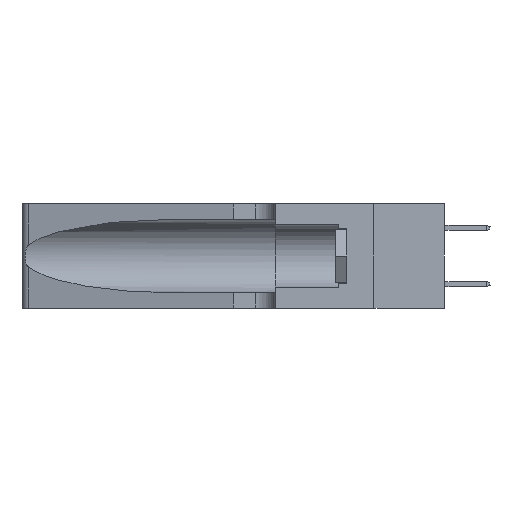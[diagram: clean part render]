
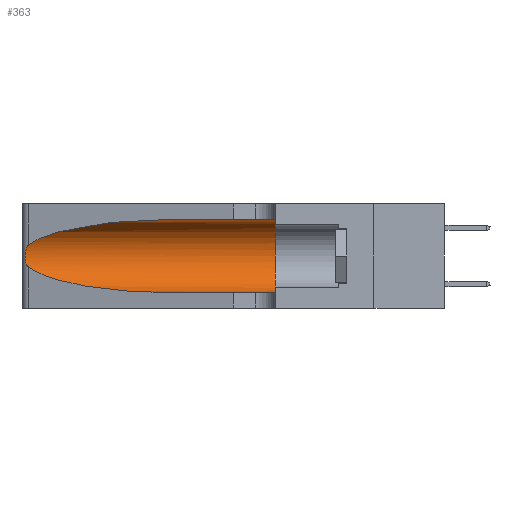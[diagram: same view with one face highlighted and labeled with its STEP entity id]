
A CAD part, left-side view. The second image highlights one B-rep face of the part: STEP entity #363.
In plain terms, the highlighted cylindrical face has radius 3.308 mm (diameter 6.617 mm), a partial arc.
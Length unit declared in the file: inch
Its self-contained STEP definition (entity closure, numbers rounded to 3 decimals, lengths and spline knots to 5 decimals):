
#363 = ADVANCED_FACE ( 'NONE', ( #7439 ), #6662, .F. ) ;
#859 = DIRECTION ( 'NONE',  ( 0., 0., -1. ) ) ;
#1838 = CARTESIAN_POINT ( 'NONE',  ( 0.26018, 1.23835, 0.19895 ) ) ;
#3108 = VERTEX_POINT ( 'NONE', #8464 ) ;
#3448 = ORIENTED_EDGE ( 'NONE', *, *, #30848, .T. ) ;
#3913 = EDGE_CURVE ( 'NONE', #27458, #19493, #26183, .T. ) ;
#4145 = CARTESIAN_POINT ( 'NONE',  ( 0.2373, 1.15595, 0.08982 ) ) ;
#4231 = ORIENTED_EDGE ( 'NONE', *, *, #16166, .T. ) ;
#4423 = CARTESIAN_POINT ( 'NONE',  ( 0.26075, 1.23896, 0.178 ) ) ;
#4663 = EDGE_LOOP ( 'NONE', ( #4231, #16134, #32386, #3448, #28124, #26350 ) ) ;
#6662 = CYLINDRICAL_SURFACE ( 'NONE', #26633, 0.13025 ) ;
#6971 = CARTESIAN_POINT ( 'NONE',  ( 0.25856, 1.23593, 0.16098 ) ) ;
#7439 = FACE_OUTER_BOUND ( 'NONE', #4663, .T. ) ;
#8286 = VERTEX_POINT ( 'NONE', #29835 ) ;
#8415 = CARTESIAN_POINT ( 'NONE',  ( 0.1305, 1.61858, 0.185 ) ) ;
#8464 = CARTESIAN_POINT ( 'NONE',  ( 0.1305, 0.35, 0.05475 ) ) ;
#8796 = DIRECTION ( 'NONE',  ( 0., -1., 0. ) ) ;
#9383 = CARTESIAN_POINT ( 'NONE',  ( 0.1305, 0.35, 0.31525 ) ) ;
#9470 = CARTESIAN_POINT ( 'NONE',  ( 0.25639, 1.23186, 0.15144 ) ) ;
#9614 = CARTESIAN_POINT ( 'NONE',  ( 0.25487, 1.22718, 0.22369 ) ) ;
#10123 = VERTEX_POINT ( 'NONE', #9614 ) ;
#11024 = VERTEX_POINT ( 'NONE', #18338 ) ;
#11747 = CARTESIAN_POINT ( 'NONE',  ( 0.18966, 0.96281, 0.31525 ) ) ;
#11996 = CARTESIAN_POINT ( 'NONE',  ( 0.25487, 1.22718, 0.14631 ) ) ;
#12451 = CARTESIAN_POINT ( 'NONE',  ( 0.1305, 0.72297, 0.31525 ) ) ;
#12587 = AXIS2_PLACEMENT_3D ( 'NONE', #30137, #15118, #25696 ) ;
#13033 = CIRCLE ( 'NONE', #12587, 0.13025 ) ;
#14299 = CARTESIAN_POINT ( 'NONE',  ( 0.18966, 0.96281, 0.05475 ) ) ;
#14415 = CARTESIAN_POINT ( 'NONE',  ( 0.2373, 1.15595, 0.28018 ) ) ;
#14455 = CARTESIAN_POINT ( 'NONE',  ( 0.25639, 1.23184, 0.21858 ) ) ;
#15118 = DIRECTION ( 'NONE',  ( 0., 1., 0. ) ) ;
#15479 = EDGE_CURVE ( 'NONE', #10123, #11024, #30214, .T. ) ;
#16045 = DIRECTION ( 'NONE',  ( 0., -1., 0. ) ) ;
#16134 = ORIENTED_EDGE ( 'NONE', *, *, #15479, .T. ) ;
#16166 = EDGE_CURVE ( 'NONE', #27458, #10123, #24427, .T. ) ;
#16916 = CARTESIAN_POINT ( 'NONE',  ( 0.25555, 1.22994, 0.2215 ) ) ;
#17024 = CARTESIAN_POINT ( 'NONE',  ( 0.25854, 1.2359, 0.20912 ) ) ;
#18064 = LINE ( 'NONE', #21408, #23979 ) ;
#18338 = CARTESIAN_POINT ( 'NONE',  ( 0.25487, 1.22718, 0.14631 ) ) ;
#18599 =( BOUNDED_CURVE ( )  B_SPLINE_CURVE ( 3, ( #21823, #4145, #14299, #31826 ),
 .UNSPECIFIED., .F., .T. ) 
 B_SPLINE_CURVE_WITH_KNOTS ( ( 4, 4 ),
 ( 3.44316, 4.71239 ),
 .UNSPECIFIED. ) 
 CURVE ( )  GEOMETRIC_REPRESENTATION_ITEM ( )  RATIONAL_B_SPLINE_CURVE ( ( 1., 0.87, 0.87, 1. ) ) 
 REPRESENTATION_ITEM ( '' )  );
#19403 = CARTESIAN_POINT ( 'NONE',  ( 0.1305, 0.72297, 0.31525 ) ) ;
#19493 = VERTEX_POINT ( 'NONE', #9383 ) ;
#19541 = CARTESIAN_POINT ( 'NONE',  ( 0.26075, 1.23896, 0.19203 ) ) ;
#20720 = EDGE_CURVE ( 'NONE', #11024, #8286, #18599, .T. ) ;
#21408 = CARTESIAN_POINT ( 'NONE',  ( 0.1305, 1.61858, 0.05475 ) ) ;
#21823 = CARTESIAN_POINT ( 'NONE',  ( 0.25487, 1.22718, 0.14631 ) ) ;
#22085 = CARTESIAN_POINT ( 'NONE',  ( 0.26017, 1.23833, 0.17102 ) ) ;
#23979 = VECTOR ( 'NONE', #8796, 39.37008 ) ;
#24427 =( BOUNDED_CURVE ( )  B_SPLINE_CURVE ( 3, ( #19403, #11747, #14415, #31953 ),
 .UNSPECIFIED., .F., .F. ) 
 B_SPLINE_CURVE_WITH_KNOTS ( ( 4, 4 ),
 ( 1.5708, 2.84003 ),
 .UNSPECIFIED. ) 
 CURVE ( )  GEOMETRIC_REPRESENTATION_ITEM ( )  RATIONAL_B_SPLINE_CURVE ( ( 1., 0.87, 0.87, 1. ) ) 
 REPRESENTATION_ITEM ( '' )  );
#24492 = CARTESIAN_POINT ( 'NONE',  ( 0.25487, 1.22718, 0.22369 ) ) ;
#24605 = CARTESIAN_POINT ( 'NONE',  ( 0.25789, 1.23486, 0.15765 ) ) ;
#25004 = EDGE_CURVE ( 'NONE', #19493, #3108, #13033, .T. ) ;
#25696 = DIRECTION ( 'NONE',  ( 0., 0., 1. ) ) ;
#26183 = LINE ( 'NONE', #26572, #32000 ) ;
#26350 = ORIENTED_EDGE ( 'NONE', *, *, #3913, .F. ) ;
#26572 = CARTESIAN_POINT ( 'NONE',  ( 0.1305, 1.61858, 0.31525 ) ) ;
#26633 = AXIS2_PLACEMENT_3D ( 'NONE', #8415, #16045, #859 ) ;
#27091 = CARTESIAN_POINT ( 'NONE',  ( 0.25555, 1.22993, 0.14849 ) ) ;
#27458 = VERTEX_POINT ( 'NONE', #12451 ) ;
#28124 = ORIENTED_EDGE ( 'NONE', *, *, #25004, .F. ) ;
#29072 = DIRECTION ( 'NONE',  ( 0., -1., 0. ) ) ;
#29835 = CARTESIAN_POINT ( 'NONE',  ( 0.1305, 0.72297, 0.05475 ) ) ;
#30137 = CARTESIAN_POINT ( 'NONE',  ( 0.1305, 0.35, 0.185 ) ) ;
#30214 = B_SPLINE_CURVE_WITH_KNOTS ( 'NONE', 3,
 ( #24492, #16916, #14455, #31990, #17024, #1838, #19541, #4423, #22085, #6971, #24605, #9470, #27091, #11996 ),
 .UNSPECIFIED., .F., .F.,
 ( 4, 2, 2, 2, 2, 2, 4 ),
 ( 0., 0.00027, 0.00053, 0.00107, 0.0016, 0.00187, 0.00214 ),
 .UNSPECIFIED. ) ;
#30848 = EDGE_CURVE ( 'NONE', #8286, #3108, #18064, .T. ) ;
#31826 = CARTESIAN_POINT ( 'NONE',  ( 0.1305, 0.72297, 0.05475 ) ) ;
#31953 = CARTESIAN_POINT ( 'NONE',  ( 0.25487, 1.22718, 0.22369 ) ) ;
#31990 = CARTESIAN_POINT ( 'NONE',  ( 0.25787, 1.23484, 0.2124 ) ) ;
#32000 = VECTOR ( 'NONE', #29072, 39.37008 ) ;
#32386 = ORIENTED_EDGE ( 'NONE', *, *, #20720, .T. ) ;
